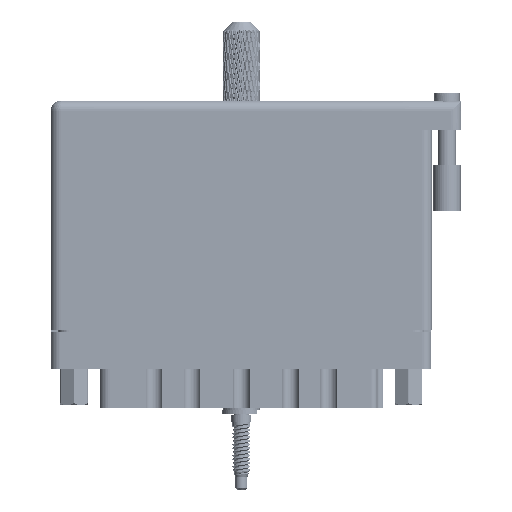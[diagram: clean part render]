
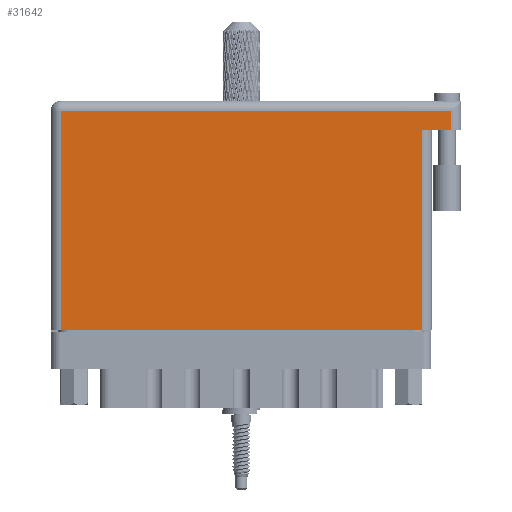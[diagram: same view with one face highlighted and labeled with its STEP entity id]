
A CAD part, front view. The second image highlights one B-rep face of the part: STEP entity #31642.
In plain terms, the highlighted face is planar.
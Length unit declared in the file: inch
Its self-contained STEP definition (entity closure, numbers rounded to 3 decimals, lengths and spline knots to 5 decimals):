
#2852 = EDGE_LOOP ( 'NONE', ( #10283, #12961, #6277, #66613, #27582, #15846 ) ) ;
#5453 = CARTESIAN_POINT ( 'NONE',  ( 0., 1.566, 0. ) ) ;
#6277 = ORIENTED_EDGE ( 'NONE', *, *, #64017, .F. ) ;
#8266 = DIRECTION ( 'NONE',  ( 1., 0., 0. ) ) ;
#10283 = ORIENTED_EDGE ( 'NONE', *, *, #59673, .T. ) ;
#12907 = CARTESIAN_POINT ( 'NONE',  ( 2.8, 1.369, 0. ) ) ;
#12961 = ORIENTED_EDGE ( 'NONE', *, *, #114678, .T. ) ;
#14574 = VECTOR ( 'NONE', #97254, 39.37008 ) ;
#15846 = ORIENTED_EDGE ( 'NONE', *, *, #98378, .T. ) ;
#17383 = CARTESIAN_POINT ( 'NONE',  ( 2.53, 1.369, 0. ) ) ;
#17990 = CARTESIAN_POINT ( 'NONE',  ( 0.07, 0., 0. ) ) ;
#21094 = CARTESIAN_POINT ( 'NONE',  ( 2.53, 1.369, 0. ) ) ;
#21146 = DIRECTION ( 'NONE',  ( -1., 0., 0. ) ) ;
#22432 = LINE ( 'NONE', #17383, #94881 ) ;
#27582 = ORIENTED_EDGE ( 'NONE', *, *, #52205, .T. ) ;
#27821 = VECTOR ( 'NONE', #81046, 39.37008 ) ;
#31642 = ADVANCED_FACE ( 'NONE', ( #44732 ), #64534, .F. ) ;
#38115 = CARTESIAN_POINT ( 'NONE',  ( 0.07, 1.496, 0. ) ) ;
#38555 = LINE ( 'NONE', #12907, #27821 ) ;
#44732 = FACE_OUTER_BOUND ( 'NONE', #2852, .T. ) ;
#45561 = VERTEX_POINT ( 'NONE', #52305 ) ;
#48903 = DIRECTION ( 'NONE',  ( 0., -1., 0. ) ) ;
#52205 = EDGE_CURVE ( 'NONE', #45561, #118216, #63204, .T. ) ;
#52305 = CARTESIAN_POINT ( 'NONE',  ( 2.73, 1.496, 0. ) ) ;
#52854 = LINE ( 'NONE', #17990, #92968 ) ;
#56633 = AXIS2_PLACEMENT_3D ( 'NONE', #5453, #103308, #74499 ) ;
#59673 = EDGE_CURVE ( 'NONE', #75940, #110400, #87220, .T. ) ;
#61211 = CARTESIAN_POINT ( 'NONE',  ( 0., 1.496, 0. ) ) ;
#63204 = LINE ( 'NONE', #61211, #126309 ) ;
#64017 = EDGE_CURVE ( 'NONE', #74704, #115930, #38555, .T. ) ;
#64534 = PLANE ( 'NONE',  #56633 ) ;
#66613 = ORIENTED_EDGE ( 'NONE', *, *, #121377, .T. ) ;
#74499 = DIRECTION ( 'NONE',  ( -1., 0., 0. ) ) ;
#74704 = VERTEX_POINT ( 'NONE', #121344 ) ;
#75940 = VERTEX_POINT ( 'NONE', #100745 ) ;
#81046 = DIRECTION ( 'NONE',  ( -1., 0., 0. ) ) ;
#87220 = LINE ( 'NONE', #96205, #102689 ) ;
#87328 = CARTESIAN_POINT ( 'NONE',  ( 2.73, 1.566, 0. ) ) ;
#92968 = VECTOR ( 'NONE', #48903, 39.37008 ) ;
#94881 = VECTOR ( 'NONE', #96651, 39.37008 ) ;
#96205 = CARTESIAN_POINT ( 'NONE',  ( 0., 0., 0. ) ) ;
#96316 = LINE ( 'NONE', #87328, #14574 ) ;
#96651 = DIRECTION ( 'NONE',  ( 0., 1., 0. ) ) ;
#97254 = DIRECTION ( 'NONE',  ( 0., 1., 0. ) ) ;
#98378 = EDGE_CURVE ( 'NONE', #118216, #75940, #52854, .T. ) ;
#100745 = CARTESIAN_POINT ( 'NONE',  ( 0.07, 0., 0. ) ) ;
#102689 = VECTOR ( 'NONE', #8266, 39.37008 ) ;
#103308 = DIRECTION ( 'NONE',  ( 0., 0., -1. ) ) ;
#110400 = VERTEX_POINT ( 'NONE', #127410 ) ;
#114678 = EDGE_CURVE ( 'NONE', #110400, #115930, #22432, .T. ) ;
#115930 = VERTEX_POINT ( 'NONE', #21094 ) ;
#118216 = VERTEX_POINT ( 'NONE', #38115 ) ;
#121344 = CARTESIAN_POINT ( 'NONE',  ( 2.73, 1.369, 0. ) ) ;
#121377 = EDGE_CURVE ( 'NONE', #74704, #45561, #96316, .T. ) ;
#126309 = VECTOR ( 'NONE', #21146, 39.37008 ) ;
#127410 = CARTESIAN_POINT ( 'NONE',  ( 2.53, 0., 0. ) ) ;
